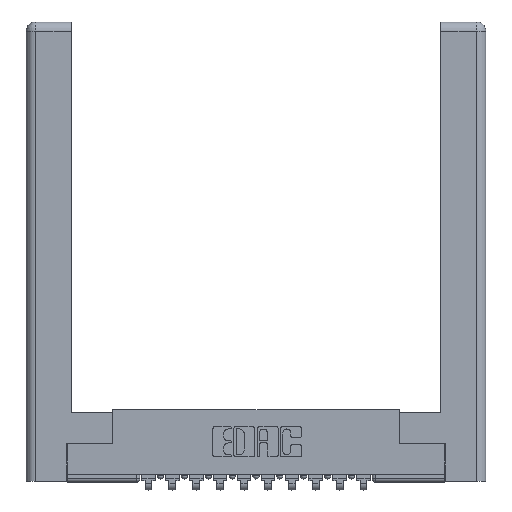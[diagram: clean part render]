
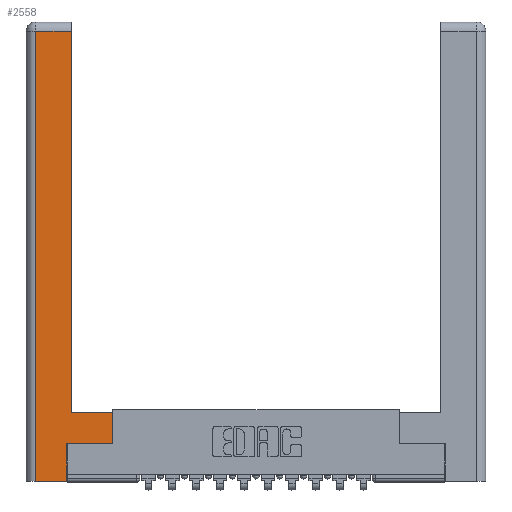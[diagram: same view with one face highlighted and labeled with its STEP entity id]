
A CAD part, top view. The second image highlights one B-rep face of the part: STEP entity #2558.
In plain terms, the highlighted planar face has unit normal (0, 0, 1).
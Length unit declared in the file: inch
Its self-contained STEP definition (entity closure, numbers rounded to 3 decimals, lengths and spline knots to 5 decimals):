
#331 = CARTESIAN_POINT ( 'NONE',  ( 0.295, 2.94, 0. ) ) ;
#452 = CARTESIAN_POINT ( 'NONE',  ( 0.265, 0.245, 0. ) ) ;
#628 = VECTOR ( 'NONE', #6267, 39.37008 ) ;
#751 = DIRECTION ( 'NONE',  ( 1., 0., 0. ) ) ;
#1416 = LINE ( 'NONE', #13620, #3850 ) ;
#1548 = VERTEX_POINT ( 'NONE', #3207 ) ;
#2012 = LINE ( 'NONE', #3563, #6654 ) ;
#2109 = CARTESIAN_POINT ( 'NONE',  ( 0.295, 0.45, 0. ) ) ;
#2179 = DIRECTION ( 'NONE',  ( 0., 1., 0. ) ) ;
#2483 = DIRECTION ( 'NONE',  ( -1., 0., 0. ) ) ;
#2558 = ADVANCED_FACE ( 'NONE', ( #7208 ), #7366, .F. ) ;
#2666 = VERTEX_POINT ( 'NONE', #4049 ) ;
#3207 = CARTESIAN_POINT ( 'NONE',  ( 0.295, 0.45, 0. ) ) ;
#3235 = VECTOR ( 'NONE', #10321, 39.37008 ) ;
#3316 = VECTOR ( 'NONE', #3986, 39.37008 ) ;
#3563 = CARTESIAN_POINT ( 'NONE',  ( 0.295, 3., 0. ) ) ;
#3651 = DIRECTION ( 'NONE',  ( 0., 0., -1. ) ) ;
#3760 = ORIENTED_EDGE ( 'NONE', *, *, #9331, .T. ) ;
#3778 = DIRECTION ( 'NONE',  ( 1., 0., 0. ) ) ;
#3850 = VECTOR ( 'NONE', #3778, 39.37008 ) ;
#3979 = VERTEX_POINT ( 'NONE', #6380 ) ;
#3986 = DIRECTION ( 'NONE',  ( 0., -1., 0. ) ) ;
#4049 = CARTESIAN_POINT ( 'NONE',  ( 0.565, 0.245, 0. ) ) ;
#4600 = EDGE_CURVE ( 'NONE', #12869, #8460, #11543, .T. ) ;
#4915 = ORIENTED_EDGE ( 'NONE', *, *, #9936, .T. ) ;
#4955 = AXIS2_PLACEMENT_3D ( 'NONE', #8410, #3651, #13501 ) ;
#4990 = LINE ( 'NONE', #7569, #14202 ) ;
#5030 = CARTESIAN_POINT ( 'NONE',  ( 0.0615, 0., 0. ) ) ;
#5153 = ORIENTED_EDGE ( 'NONE', *, *, #11151, .T. ) ;
#5253 = EDGE_CURVE ( 'NONE', #2666, #3979, #14790, .T. ) ;
#5568 = ORIENTED_EDGE ( 'NONE', *, *, #4600, .T. ) ;
#5910 = DIRECTION ( 'NONE',  ( -1., 0., 0. ) ) ;
#6162 = VERTEX_POINT ( 'NONE', #7139 ) ;
#6267 = DIRECTION ( 'NONE',  ( 0., 1., 0. ) ) ;
#6380 = CARTESIAN_POINT ( 'NONE',  ( 0.565, 0.45, 0. ) ) ;
#6654 = VECTOR ( 'NONE', #2179, 39.37008 ) ;
#7139 = CARTESIAN_POINT ( 'NONE',  ( 0.0615, 0., 0. ) ) ;
#7208 = FACE_OUTER_BOUND ( 'NONE', #9459, .T. ) ;
#7366 = PLANE ( 'NONE',  #4955 ) ;
#7569 = CARTESIAN_POINT ( 'NONE',  ( 0.0615, 2.94, 0. ) ) ;
#7941 = ORIENTED_EDGE ( 'NONE', *, *, #9083, .T. ) ;
#8353 = LINE ( 'NONE', #14451, #11401 ) ;
#8410 = CARTESIAN_POINT ( 'NONE',  ( 0., 0., 0. ) ) ;
#8460 = VERTEX_POINT ( 'NONE', #15198 ) ;
#8985 = EDGE_CURVE ( 'NONE', #3979, #1548, #11010, .T. ) ;
#9083 = EDGE_CURVE ( 'NONE', #14204, #6162, #13826, .T. ) ;
#9331 = EDGE_CURVE ( 'NONE', #1548, #12275, #2012, .T. ) ;
#9459 = EDGE_LOOP ( 'NONE', ( #3760, #5153, #7941, #4915, #5568, #12903, #10340, #14550 ) ) ;
#9936 = EDGE_CURVE ( 'NONE', #6162, #12869, #1416, .T. ) ;
#9993 = CARTESIAN_POINT ( 'NONE',  ( 0.565, 0.45, 0. ) ) ;
#10321 = DIRECTION ( 'NONE',  ( 0., 1., 0. ) ) ;
#10340 = ORIENTED_EDGE ( 'NONE', *, *, #5253, .T. ) ;
#10475 = CARTESIAN_POINT ( 'NONE',  ( 0.0615, 2.94, 0. ) ) ;
#11010 = LINE ( 'NONE', #2109, #12061 ) ;
#11151 = EDGE_CURVE ( 'NONE', #12275, #14204, #4990, .T. ) ;
#11401 = VECTOR ( 'NONE', #751, 39.37008 ) ;
#11543 = LINE ( 'NONE', #452, #3235 ) ;
#12061 = VECTOR ( 'NONE', #5910, 39.37008 ) ;
#12275 = VERTEX_POINT ( 'NONE', #331 ) ;
#12869 = VERTEX_POINT ( 'NONE', #15404 ) ;
#12903 = ORIENTED_EDGE ( 'NONE', *, *, #13140, .T. ) ;
#13140 = EDGE_CURVE ( 'NONE', #8460, #2666, #8353, .T. ) ;
#13501 = DIRECTION ( 'NONE',  ( -1., 0., 0. ) ) ;
#13620 = CARTESIAN_POINT ( 'NONE',  ( 0.265, 0., 0. ) ) ;
#13826 = LINE ( 'NONE', #5030, #3316 ) ;
#14202 = VECTOR ( 'NONE', #2483, 39.37008 ) ;
#14204 = VERTEX_POINT ( 'NONE', #10475 ) ;
#14451 = CARTESIAN_POINT ( 'NONE',  ( 0.565, 0.245, 0. ) ) ;
#14550 = ORIENTED_EDGE ( 'NONE', *, *, #8985, .T. ) ;
#14790 = LINE ( 'NONE', #9993, #628 ) ;
#15198 = CARTESIAN_POINT ( 'NONE',  ( 0.265, 0.245, 0. ) ) ;
#15404 = CARTESIAN_POINT ( 'NONE',  ( 0.265, 0., 0. ) ) ;
